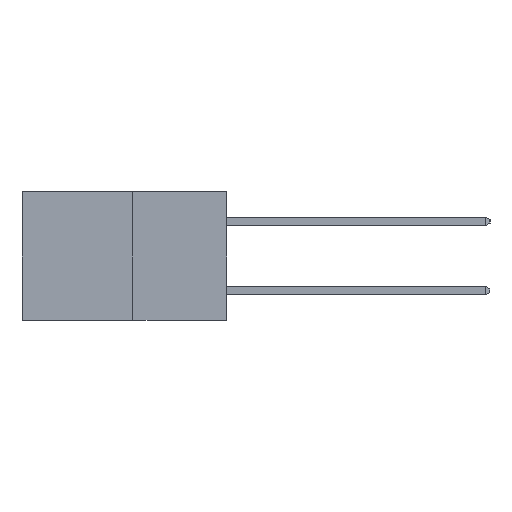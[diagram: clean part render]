
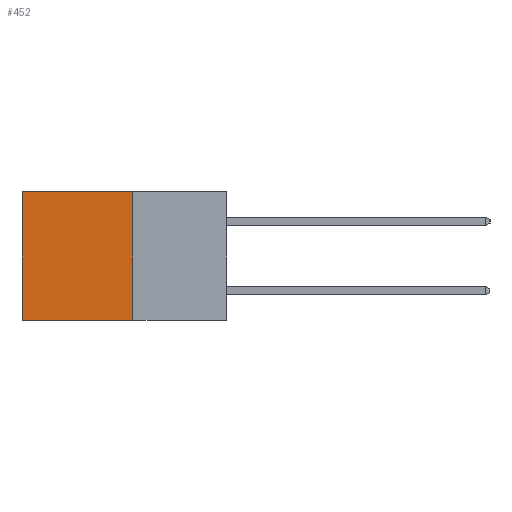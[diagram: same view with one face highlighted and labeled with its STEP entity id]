
A CAD part, left-side view. The second image highlights one B-rep face of the part: STEP entity #452.
In plain terms, the highlighted planar face has unit normal (-1, 0, 0).
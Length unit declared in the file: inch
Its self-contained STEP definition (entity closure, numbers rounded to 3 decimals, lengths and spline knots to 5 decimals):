
#452 = ADVANCED_FACE ( 'NONE', ( #11499 ), #13776, .F. ) ;
#541 = EDGE_CURVE ( 'NONE', #20734, #6690, #13923, .T. ) ;
#1305 = VECTOR ( 'NONE', #16247, 39.37008 ) ;
#1659 = VECTOR ( 'NONE', #6083, 39.37008 ) ;
#2212 = CARTESIAN_POINT ( 'NONE',  ( 0.277, 0.27, -0.37 ) ) ;
#2314 = DIRECTION ( 'NONE',  ( 1., 0., 0. ) ) ;
#2964 = DIRECTION ( 'NONE',  ( 0., 0., -1. ) ) ;
#3552 = VECTOR ( 'NONE', #8496, 39.37008 ) ;
#4005 = AXIS2_PLACEMENT_3D ( 'NONE', #2212, #2314, #15555 ) ;
#4975 = ORIENTED_EDGE ( 'NONE', *, *, #12943, .F. ) ;
#6083 = DIRECTION ( 'NONE',  ( 0., 0., -1. ) ) ;
#6295 = ORIENTED_EDGE ( 'NONE', *, *, #17716, .F. ) ;
#6491 = CARTESIAN_POINT ( 'NONE',  ( 0.277, 0.27, 0. ) ) ;
#6564 = CARTESIAN_POINT ( 'NONE',  ( 0.277, 0.59, -0.37 ) ) ;
#6690 = VERTEX_POINT ( 'NONE', #18121 ) ;
#7320 = ORIENTED_EDGE ( 'NONE', *, *, #541, .T. ) ;
#8248 = VERTEX_POINT ( 'NONE', #6491 ) ;
#8496 = DIRECTION ( 'NONE',  ( 0., 1., 0. ) ) ;
#11499 = FACE_OUTER_BOUND ( 'NONE', #22264, .T. ) ;
#11621 = CARTESIAN_POINT ( 'NONE',  ( 0.277, 0.27, -0.37 ) ) ;
#11628 = CARTESIAN_POINT ( 'NONE',  ( 0.277, 0.27, -0.37 ) ) ;
#12577 = ORIENTED_EDGE ( 'NONE', *, *, #17342, .T. ) ;
#12943 = EDGE_CURVE ( 'NONE', #8248, #14933, #17461, .T. ) ;
#13776 = PLANE ( 'NONE',  #4005 ) ;
#13923 = LINE ( 'NONE', #6564, #1659 ) ;
#14513 = CARTESIAN_POINT ( 'NONE',  ( 0.277, 0.27, 0. ) ) ;
#14933 = VERTEX_POINT ( 'NONE', #11621 ) ;
#15163 = LINE ( 'NONE', #14513, #1305 ) ;
#15555 = DIRECTION ( 'NONE',  ( 0., 0., -1. ) ) ;
#16247 = DIRECTION ( 'NONE',  ( 0., 1., 0. ) ) ;
#17342 = EDGE_CURVE ( 'NONE', #8248, #20734, #15163, .T. ) ;
#17461 = LINE ( 'NONE', #11628, #21519 ) ;
#17716 = EDGE_CURVE ( 'NONE', #14933, #6690, #21378, .T. ) ;
#18121 = CARTESIAN_POINT ( 'NONE',  ( 0.277, 0.59, -0.37 ) ) ;
#20734 = VERTEX_POINT ( 'NONE', #22019 ) ;
#20833 = CARTESIAN_POINT ( 'NONE',  ( 0.277, 0.27, -0.37 ) ) ;
#21378 = LINE ( 'NONE', #20833, #3552 ) ;
#21519 = VECTOR ( 'NONE', #2964, 39.37008 ) ;
#22019 = CARTESIAN_POINT ( 'NONE',  ( 0.277, 0.59, 0. ) ) ;
#22264 = EDGE_LOOP ( 'NONE', ( #7320, #6295, #4975, #12577 ) ) ;
